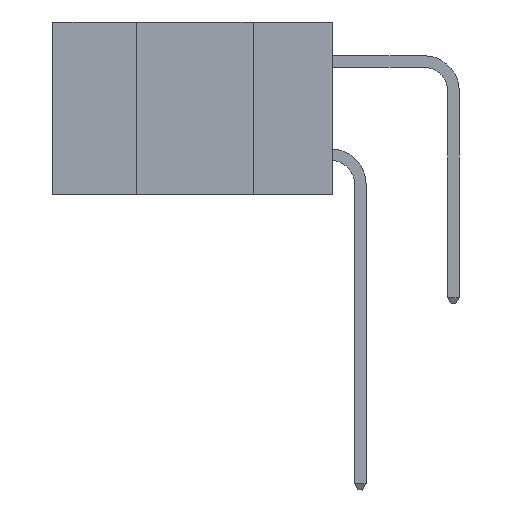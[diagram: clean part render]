
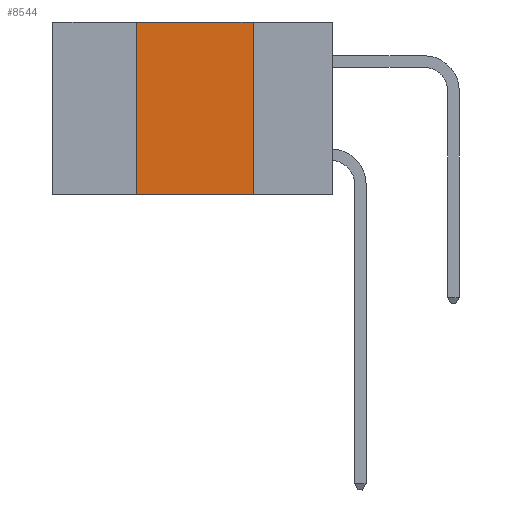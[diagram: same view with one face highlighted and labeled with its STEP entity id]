
A CAD part, left-side view. The second image highlights one B-rep face of the part: STEP entity #8544.
In plain terms, the highlighted planar face has unit normal (-1, 0, 0).
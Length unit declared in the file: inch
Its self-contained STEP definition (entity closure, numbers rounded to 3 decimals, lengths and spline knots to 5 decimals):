
#21 = EDGE_CURVE ( 'NONE', #10540, #6153, #2747, .T. ) ;
#639 = ORIENTED_EDGE ( 'NONE', *, *, #3361, .F. ) ;
#1086 = LINE ( 'NONE', #8532, #1875 ) ;
#1875 = VECTOR ( 'NONE', #10374, 39.37008 ) ;
#1887 = CARTESIAN_POINT ( 'NONE',  ( 0., 0.42, -0.37 ) ) ;
#1962 = CARTESIAN_POINT ( 'NONE',  ( 0., 0.17, -0.37 ) ) ;
#2089 = LINE ( 'NONE', #1962, #2569 ) ;
#2569 = VECTOR ( 'NONE', #5724, 39.37008 ) ;
#2732 = CARTESIAN_POINT ( 'NONE',  ( 0., 0.6, 0. ) ) ;
#2747 = LINE ( 'NONE', #1887, #11481 ) ;
#2817 = EDGE_CURVE ( 'NONE', #9906, #5244, #2089, .T. ) ;
#3361 = EDGE_CURVE ( 'NONE', #6153, #9906, #11961, .T. ) ;
#3470 = PLANE ( 'NONE',  #12090 ) ;
#3792 = DIRECTION ( 'NONE',  ( 0., 0., 1. ) ) ;
#4208 = DIRECTION ( 'NONE',  ( 0., 0., -1. ) ) ;
#4694 = DIRECTION ( 'NONE',  ( 0., -1., 0. ) ) ;
#4744 = VECTOR ( 'NONE', #4694, 39.37008 ) ;
#5244 = VERTEX_POINT ( 'NONE', #8857 ) ;
#5724 = DIRECTION ( 'NONE',  ( 0., 0., -1. ) ) ;
#6128 = DIRECTION ( 'NONE',  ( 1., 0., 0. ) ) ;
#6153 = VERTEX_POINT ( 'NONE', #9355 ) ;
#7078 = EDGE_LOOP ( 'NONE', ( #10682, #639, #10319, #9183 ) ) ;
#7124 = CARTESIAN_POINT ( 'NONE',  ( 0., 0.17, 0. ) ) ;
#7227 = FACE_OUTER_BOUND ( 'NONE', #7078, .T. ) ;
#7275 = EDGE_CURVE ( 'NONE', #10540, #5244, #1086, .T. ) ;
#8532 = CARTESIAN_POINT ( 'NONE',  ( 0., 0.6, -0.37 ) ) ;
#8544 = ADVANCED_FACE ( 'NONE', ( #7227 ), #3470, .F. ) ;
#8857 = CARTESIAN_POINT ( 'NONE',  ( 0., 0.17, -0.37 ) ) ;
#9183 = ORIENTED_EDGE ( 'NONE', *, *, #7275, .T. ) ;
#9355 = CARTESIAN_POINT ( 'NONE',  ( 0., 0.42, 0. ) ) ;
#9906 = VERTEX_POINT ( 'NONE', #7124 ) ;
#10319 = ORIENTED_EDGE ( 'NONE', *, *, #21, .F. ) ;
#10374 = DIRECTION ( 'NONE',  ( 0., -1., 0. ) ) ;
#10540 = VERTEX_POINT ( 'NONE', #12004 ) ;
#10682 = ORIENTED_EDGE ( 'NONE', *, *, #2817, .F. ) ;
#10849 = CARTESIAN_POINT ( 'NONE',  ( 0., 0.6, 0. ) ) ;
#11481 = VECTOR ( 'NONE', #3792, 39.37008 ) ;
#11961 = LINE ( 'NONE', #2732, #4744 ) ;
#12004 = CARTESIAN_POINT ( 'NONE',  ( 0., 0.42, -0.37 ) ) ;
#12090 = AXIS2_PLACEMENT_3D ( 'NONE', #10849, #6128, #4208 ) ;
